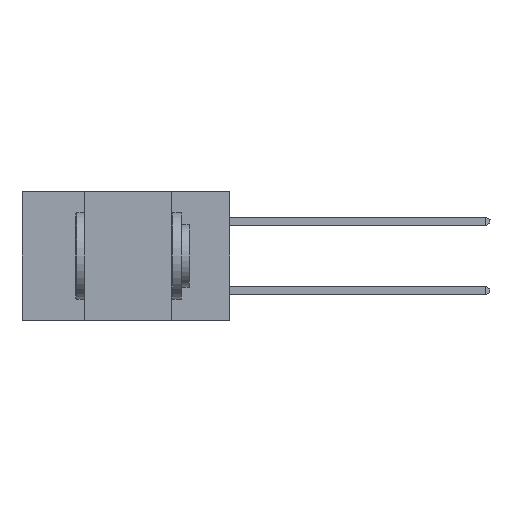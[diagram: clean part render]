
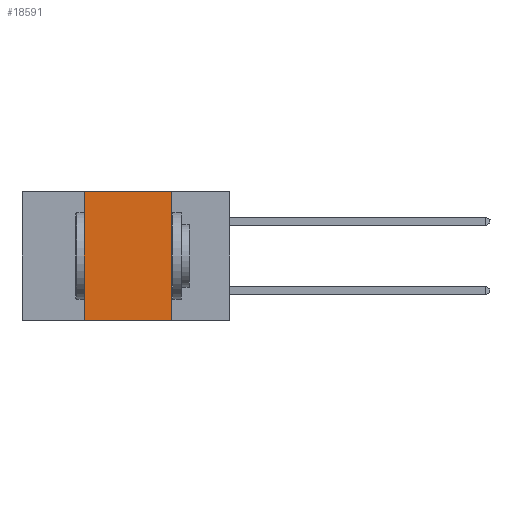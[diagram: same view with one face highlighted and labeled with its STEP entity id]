
A CAD part, left-side view. The second image highlights one B-rep face of the part: STEP entity #18591.
In plain terms, the highlighted planar face has unit normal (-1, 0, 0).
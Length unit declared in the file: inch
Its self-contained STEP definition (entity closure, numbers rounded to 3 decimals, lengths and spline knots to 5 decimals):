
#562 = DIRECTION ( 'NONE',  ( 0., 0., -1. ) ) ;
#579 = DIRECTION ( 'NONE',  ( 0., 0., -1. ) ) ;
#678 = EDGE_CURVE ( 'NONE', #7504, #6243, #16792, .T. ) ;
#1356 = VECTOR ( 'NONE', #562, 39.37008 ) ;
#1916 = CARTESIAN_POINT ( 'NONE',  ( 0., 0.6, -0.37 ) ) ;
#2209 = DIRECTION ( 'NONE',  ( 1., 0., 0. ) ) ;
#2306 = CARTESIAN_POINT ( 'NONE',  ( 0., 0.17, -0.37 ) ) ;
#3816 = PLANE ( 'NONE',  #5338 ) ;
#5338 = AXIS2_PLACEMENT_3D ( 'NONE', #16911, #2209, #579 ) ;
#5652 = FACE_OUTER_BOUND ( 'NONE', #6437, .T. ) ;
#5853 = CARTESIAN_POINT ( 'NONE',  ( 0., 0.42, 0. ) ) ;
#5869 = DIRECTION ( 'NONE',  ( 0., -1., 0. ) ) ;
#5893 = ORIENTED_EDGE ( 'NONE', *, *, #678, .F. ) ;
#6057 = EDGE_CURVE ( 'NONE', #14919, #7504, #16078, .T. ) ;
#6243 = VERTEX_POINT ( 'NONE', #18200 ) ;
#6437 = EDGE_LOOP ( 'NONE', ( #5893, #18780, #14147, #18614 ) ) ;
#6527 = VECTOR ( 'NONE', #5869, 39.37008 ) ;
#7383 = VECTOR ( 'NONE', #17572, 39.37008 ) ;
#7504 = VERTEX_POINT ( 'NONE', #14996 ) ;
#7591 = CARTESIAN_POINT ( 'NONE',  ( 0., 0.42, -0.37 ) ) ;
#9415 = CARTESIAN_POINT ( 'NONE',  ( 0., 0.42, -0.37 ) ) ;
#9740 = CARTESIAN_POINT ( 'NONE',  ( 0., 0.6, 0. ) ) ;
#10408 = EDGE_CURVE ( 'NONE', #19664, #6243, #18524, .T. ) ;
#14147 = ORIENTED_EDGE ( 'NONE', *, *, #16785, .F. ) ;
#14919 = VERTEX_POINT ( 'NONE', #5853 ) ;
#14996 = CARTESIAN_POINT ( 'NONE',  ( 0., 0.17, 0. ) ) ;
#16078 = LINE ( 'NONE', #9740, #19572 ) ;
#16785 = EDGE_CURVE ( 'NONE', #19664, #14919, #17353, .T. ) ;
#16792 = LINE ( 'NONE', #2306, #1356 ) ;
#16911 = CARTESIAN_POINT ( 'NONE',  ( 0., 0.6, 0. ) ) ;
#17353 = LINE ( 'NONE', #7591, #7383 ) ;
#17572 = DIRECTION ( 'NONE',  ( 0., 0., 1. ) ) ;
#17681 = DIRECTION ( 'NONE',  ( 0., -1., 0. ) ) ;
#18200 = CARTESIAN_POINT ( 'NONE',  ( 0., 0.17, -0.37 ) ) ;
#18524 = LINE ( 'NONE', #1916, #6527 ) ;
#18591 = ADVANCED_FACE ( 'NONE', ( #5652 ), #3816, .F. ) ;
#18614 = ORIENTED_EDGE ( 'NONE', *, *, #10408, .T. ) ;
#18780 = ORIENTED_EDGE ( 'NONE', *, *, #6057, .F. ) ;
#19572 = VECTOR ( 'NONE', #17681, 39.37008 ) ;
#19664 = VERTEX_POINT ( 'NONE', #9415 ) ;
